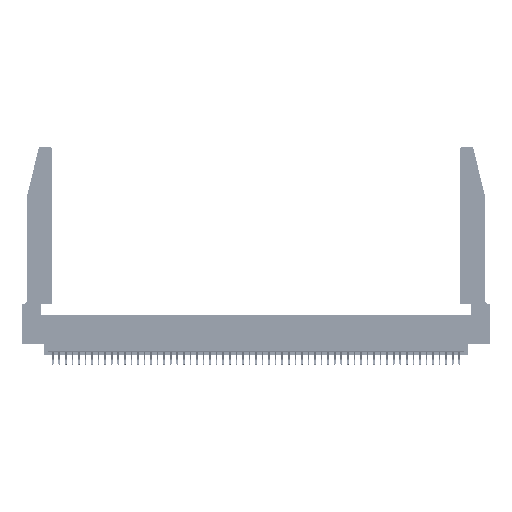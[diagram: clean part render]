
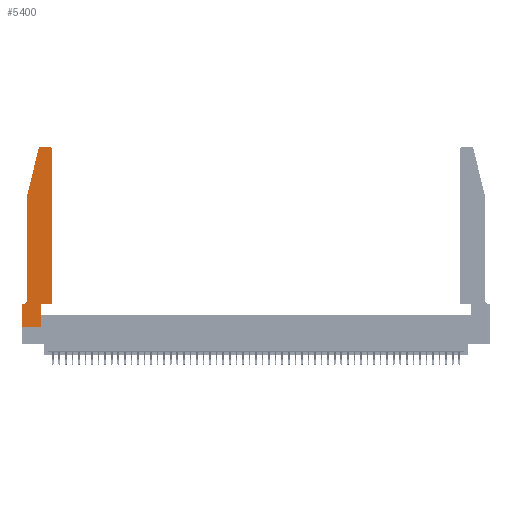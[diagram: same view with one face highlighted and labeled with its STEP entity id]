
A CAD part, top view. The second image highlights one B-rep face of the part: STEP entity #5400.
In plain terms, the highlighted planar face has unit normal (0, 0, 1).
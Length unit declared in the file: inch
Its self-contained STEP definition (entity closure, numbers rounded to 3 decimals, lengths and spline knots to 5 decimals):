
#192 = ORIENTED_EDGE ( 'NONE', *, *, #25711, .T. ) ;
#238 = ORIENTED_EDGE ( 'NONE', *, *, #15500, .T. ) ;
#859 = VECTOR ( 'NONE', #32595, 39.37008 ) ;
#1629 = LINE ( 'NONE', #31570, #32451 ) ;
#2651 = CARTESIAN_POINT ( 'NONE',  ( 0.0055, 0.35, 0.37 ) ) ;
#3405 = LINE ( 'NONE', #44503, #859 ) ;
#3494 = CARTESIAN_POINT ( 'NONE',  ( 0.0755, 0.35, 0.37 ) ) ;
#3715 = DIRECTION ( 'NONE',  ( 1., 0., 0. ) ) ;
#4499 = EDGE_CURVE ( 'NONE', #26130, #31815, #10535, .T. ) ;
#5103 = ORIENTED_EDGE ( 'NONE', *, *, #29820, .T. ) ;
#5400 = ADVANCED_FACE ( 'NONE', ( #6919 ), #30921, .T. ) ;
#5501 = CARTESIAN_POINT ( 'NONE',  ( 0.0755, 2., 0.37 ) ) ;
#5693 = CARTESIAN_POINT ( 'NONE',  ( 0.2865, 0.35, 0.37 ) ) ;
#6301 = VERTEX_POINT ( 'NONE', #37028 ) ;
#6769 = DIRECTION ( 'NONE',  ( -1., 0., 0. ) ) ;
#6821 = CARTESIAN_POINT ( 'NONE',  ( 0., 0.35, 0.37 ) ) ;
#6919 = FACE_OUTER_BOUND ( 'NONE', #51479, .T. ) ;
#7389 = CARTESIAN_POINT ( 'NONE',  ( 0.0755, 0.42, 0.37 ) ) ;
#7463 = AXIS2_PLACEMENT_3D ( 'NONE', #6821, #34870, #10869 ) ;
#7548 = DIRECTION ( 'NONE',  ( -1., 0., 0. ) ) ;
#7732 = LINE ( 'NONE', #34812, #29131 ) ;
#8617 = AXIS2_PLACEMENT_3D ( 'NONE', #42258, #18486, #46239 ) ;
#8886 = DIRECTION ( 'NONE',  ( 1., 0., 0. ) ) ;
#9733 = DIRECTION ( 'NONE',  ( 0., 1., 0. ) ) ;
#9766 = CIRCLE ( 'NONE', #47240, 0.03 ) ;
#10535 = LINE ( 'NONE', #30117, #30677 ) ;
#10869 = DIRECTION ( 'NONE',  ( 1., 0., 0. ) ) ;
#10883 = DIRECTION ( 'NONE',  ( 0., 1., 0. ) ) ;
#11188 = CARTESIAN_POINT ( 'NONE',  ( 0.0755, 2., 0.37 ) ) ;
#11360 = CARTESIAN_POINT ( 'NONE',  ( 0., 0., 0.37 ) ) ;
#11419 = VERTEX_POINT ( 'NONE', #17152 ) ;
#14026 = VECTOR ( 'NONE', #10883, 39.37008 ) ;
#15471 = AXIS2_PLACEMENT_3D ( 'NONE', #18441, #46205, #22474 ) ;
#15500 = EDGE_CURVE ( 'NONE', #43901, #43108, #9766, .T. ) ;
#17152 = CARTESIAN_POINT ( 'NONE',  ( 0.2865, 0.35, 0.37 ) ) ;
#17889 = LINE ( 'NONE', #5501, #47055 ) ;
#18196 = VECTOR ( 'NONE', #9733, 39.37008 ) ;
#18441 = CARTESIAN_POINT ( 'NONE',  ( 0.0055, 0.42, 0.37 ) ) ;
#18486 = DIRECTION ( 'NONE',  ( 0., 0., 1. ) ) ;
#18539 = EDGE_CURVE ( 'NONE', #36438, #43901, #24702, .T. ) ;
#18578 = VERTEX_POINT ( 'NONE', #27077 ) ;
#19453 = LINE ( 'NONE', #5693, #18196 ) ;
#19703 = DIRECTION ( 'NONE',  ( 0., -1., 0. ) ) ;
#20541 = ORIENTED_EDGE ( 'NONE', *, *, #44521, .T. ) ;
#21274 = ORIENTED_EDGE ( 'NONE', *, *, #18539, .T. ) ;
#22441 = VERTEX_POINT ( 'NONE', #2651 ) ;
#22474 = DIRECTION ( 'NONE',  ( -1., 0., 0. ) ) ;
#22475 = ORIENTED_EDGE ( 'NONE', *, *, #37063, .T. ) ;
#23740 = VERTEX_POINT ( 'NONE', #11360 ) ;
#24702 = LINE ( 'NONE', #34884, #14026 ) ;
#25400 = DIRECTION ( 'NONE',  ( 0., -1., 0. ) ) ;
#25711 = EDGE_CURVE ( 'NONE', #18578, #11419, #19453, .T. ) ;
#25779 = EDGE_CURVE ( 'NONE', #37793, #22441, #39296, .T. ) ;
#26108 = DIRECTION ( 'NONE',  ( -0.239, -0.971, 0. ) ) ;
#26130 = VERTEX_POINT ( 'NONE', #32358 ) ;
#27077 = CARTESIAN_POINT ( 'NONE',  ( 0.2865, 0., 0.37 ) ) ;
#27224 = EDGE_CURVE ( 'NONE', #6301, #23740, #1629, .T. ) ;
#27819 = DIRECTION ( 'NONE',  ( 0., 0., 1. ) ) ;
#28015 = CARTESIAN_POINT ( 'NONE',  ( 0.4205, 2.75, 0.37 ) ) ;
#29131 = VECTOR ( 'NONE', #6769, 39.37008 ) ;
#29148 = CARTESIAN_POINT ( 'NONE',  ( 0.4505, 2.72, 0.37 ) ) ;
#29820 = EDGE_CURVE ( 'NONE', #22441, #6301, #31563, .T. ) ;
#30117 = CARTESIAN_POINT ( 'NONE',  ( 0.0755, 2., 0.37 ) ) ;
#30677 = VECTOR ( 'NONE', #26108, 39.37008 ) ;
#30921 = PLANE ( 'NONE',  #7463 ) ;
#31248 = CARTESIAN_POINT ( 'NONE',  ( 0.284, 2.75, 0.37 ) ) ;
#31563 = LINE ( 'NONE', #3494, #51314 ) ;
#31570 = CARTESIAN_POINT ( 'NONE',  ( 0., 0., 0.37 ) ) ;
#31815 = VERTEX_POINT ( 'NONE', #11188 ) ;
#32358 = CARTESIAN_POINT ( 'NONE',  ( 0.25487, 2.72718, 0.37 ) ) ;
#32451 = VECTOR ( 'NONE', #19703, 39.37008 ) ;
#32595 = DIRECTION ( 'NONE',  ( 1., 0., 0. ) ) ;
#33191 = ORIENTED_EDGE ( 'NONE', *, *, #35956, .T. ) ;
#34812 = CARTESIAN_POINT ( 'NONE',  ( 0.2605, 2.75, 0.37 ) ) ;
#34870 = DIRECTION ( 'NONE',  ( 0., 0., 1. ) ) ;
#34884 = CARTESIAN_POINT ( 'NONE',  ( 0.4505, 0.35, 0.37 ) ) ;
#35321 = ORIENTED_EDGE ( 'NONE', *, *, #27224, .T. ) ;
#35448 = CIRCLE ( 'NONE', #8617, 0.03 ) ;
#35956 = EDGE_CURVE ( 'NONE', #46119, #26130, #35448, .T. ) ;
#36438 = VERTEX_POINT ( 'NONE', #42571 ) ;
#37028 = CARTESIAN_POINT ( 'NONE',  ( 0., 0.35, 0.37 ) ) ;
#37063 = EDGE_CURVE ( 'NONE', #43108, #46119, #7732, .T. ) ;
#37312 = ORIENTED_EDGE ( 'NONE', *, *, #25779, .T. ) ;
#37474 = EDGE_CURVE ( 'NONE', #31815, #37793, #17889, .T. ) ;
#37519 = VECTOR ( 'NONE', #8886, 39.37008 ) ;
#37793 = VERTEX_POINT ( 'NONE', #7389 ) ;
#39296 = CIRCLE ( 'NONE', #15471, 0.07 ) ;
#39989 = LINE ( 'NONE', #44873, #37519 ) ;
#42258 = CARTESIAN_POINT ( 'NONE',  ( 0.284, 2.72, 0.37 ) ) ;
#42571 = CARTESIAN_POINT ( 'NONE',  ( 0.4505, 0.35, 0.37 ) ) ;
#43108 = VERTEX_POINT ( 'NONE', #28015 ) ;
#43713 = ORIENTED_EDGE ( 'NONE', *, *, #48667, .T. ) ;
#43901 = VERTEX_POINT ( 'NONE', #29148 ) ;
#44503 = CARTESIAN_POINT ( 'NONE',  ( 0.4505, 0.35, 0.37 ) ) ;
#44521 = EDGE_CURVE ( 'NONE', #11419, #36438, #3405, .T. ) ;
#44873 = CARTESIAN_POINT ( 'NONE',  ( 0., 0., 0.37 ) ) ;
#46119 = VERTEX_POINT ( 'NONE', #31248 ) ;
#46205 = DIRECTION ( 'NONE',  ( 0., 0., -1. ) ) ;
#46239 = DIRECTION ( 'NONE',  ( 1., 0., 0. ) ) ;
#47055 = VECTOR ( 'NONE', #25400, 39.37008 ) ;
#47240 = AXIS2_PLACEMENT_3D ( 'NONE', #51501, #27819, #3715 ) ;
#47793 = ORIENTED_EDGE ( 'NONE', *, *, #37474, .T. ) ;
#48667 = EDGE_CURVE ( 'NONE', #23740, #18578, #39989, .T. ) ;
#49470 = ORIENTED_EDGE ( 'NONE', *, *, #4499, .T. ) ;
#51314 = VECTOR ( 'NONE', #7548, 39.37008 ) ;
#51479 = EDGE_LOOP ( 'NONE', ( #22475, #33191, #49470, #47793, #37312, #5103, #35321, #43713, #192, #20541, #21274, #238 ) ) ;
#51501 = CARTESIAN_POINT ( 'NONE',  ( 0.4205, 2.72, 0.37 ) ) ;
